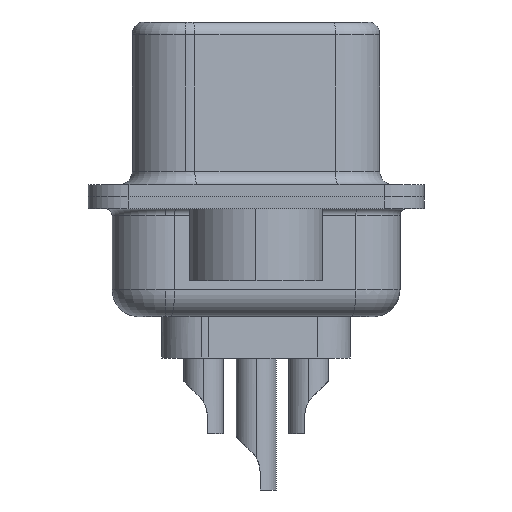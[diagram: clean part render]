
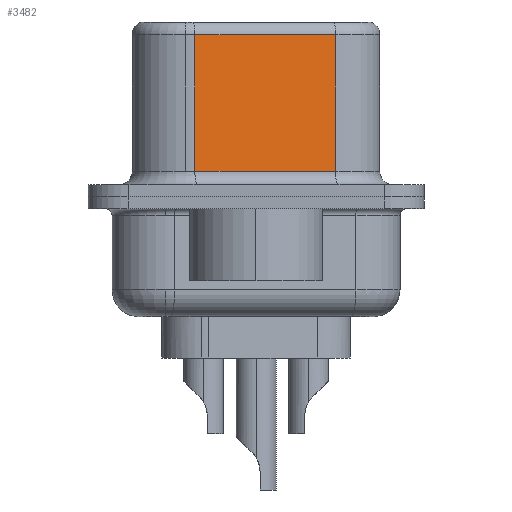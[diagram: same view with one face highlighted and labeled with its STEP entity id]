
A CAD part, left-side view. The second image highlights one B-rep face of the part: STEP entity #3482.
In plain terms, the highlighted planar face has unit normal (-0.985, -0.174, 0).
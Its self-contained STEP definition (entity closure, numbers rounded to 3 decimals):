
#156 = LINE ( 'NONE', #3406, #8589 ) ;
#806 = CARTESIAN_POINT ( 'NONE',  ( 4.546, -2.987, 0.95 ) ) ;
#1455 = VERTEX_POINT ( 'NONE', #9999 ) ;
#1708 = FACE_OUTER_BOUND ( 'NONE', #10044, .T. ) ;
#1802 = DIRECTION ( 'NONE',  ( 0.985, 0.174, 0. ) ) ;
#3406 = CARTESIAN_POINT ( 'NONE',  ( 4.546, -2.987, 6.57 ) ) ;
#3465 = CARTESIAN_POINT ( 'NONE',  ( 4.546, -2.987, 6.07 ) ) ;
#3482 = ADVANCED_FACE ( 'NONE', ( #1708 ), #13940, .F. ) ;
#3690 = VERTEX_POINT ( 'NONE', #3465 ) ;
#4228 = LINE ( 'NONE', #16386, #4256 ) ;
#4256 = VECTOR ( 'NONE', #9318, 1000. ) ;
#4420 = EDGE_CURVE ( 'NONE', #17176, #1455, #10435, .T. ) ;
#5634 = CARTESIAN_POINT ( 'NONE',  ( 3.615, 2.293, 6.07 ) ) ;
#7024 = CARTESIAN_POINT ( 'NONE',  ( 4.546, -2.987, 6.07 ) ) ;
#8589 = VECTOR ( 'NONE', #15545, 1000. ) ;
#9316 = CARTESIAN_POINT ( 'NONE',  ( 3.615, 2.293, 6.57 ) ) ;
#9318 = DIRECTION ( 'NONE',  ( 0.174, -0.985, 0. ) ) ;
#9999 = CARTESIAN_POINT ( 'NONE',  ( 3.615, 2.293, 0.95 ) ) ;
#10044 = EDGE_LOOP ( 'NONE', ( #14452, #17179, #16745, #13637 ) ) ;
#10170 = VECTOR ( 'NONE', #17577, 1000. ) ;
#10435 = LINE ( 'NONE', #9316, #11237 ) ;
#11237 = VECTOR ( 'NONE', #16487, 1000. ) ;
#13637 = ORIENTED_EDGE ( 'NONE', *, *, #18724, .T. ) ;
#13644 = CARTESIAN_POINT ( 'NONE',  ( 4.546, -2.987, 6.57 ) ) ;
#13940 = PLANE ( 'NONE',  #19298 ) ;
#14452 = ORIENTED_EDGE ( 'NONE', *, *, #15976, .F. ) ;
#14698 = VERTEX_POINT ( 'NONE', #806 ) ;
#15124 = EDGE_CURVE ( 'NONE', #3690, #17176, #19152, .T. ) ;
#15231 = DIRECTION ( 'NONE',  ( -0.174, 0.985, 0. ) ) ;
#15545 = DIRECTION ( 'NONE',  ( 0., 0., -1. ) ) ;
#15976 = EDGE_CURVE ( 'NONE', #3690, #14698, #156, .T. ) ;
#16386 = CARTESIAN_POINT ( 'NONE',  ( 4.546, -2.987, 0.95 ) ) ;
#16487 = DIRECTION ( 'NONE',  ( 0., 0., -1. ) ) ;
#16745 = ORIENTED_EDGE ( 'NONE', *, *, #4420, .T. ) ;
#17176 = VERTEX_POINT ( 'NONE', #5634 ) ;
#17179 = ORIENTED_EDGE ( 'NONE', *, *, #15124, .T. ) ;
#17577 = DIRECTION ( 'NONE',  ( -0.174, 0.985, 0. ) ) ;
#18724 = EDGE_CURVE ( 'NONE', #1455, #14698, #4228, .T. ) ;
#19152 = LINE ( 'NONE', #7024, #10170 ) ;
#19298 = AXIS2_PLACEMENT_3D ( 'NONE', #13644, #1802, #15231 ) ;
